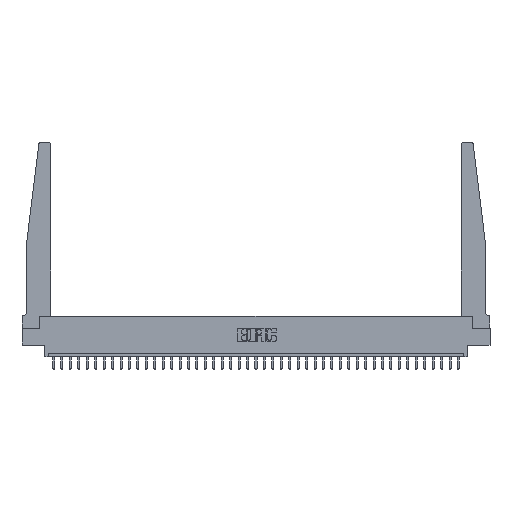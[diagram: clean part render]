
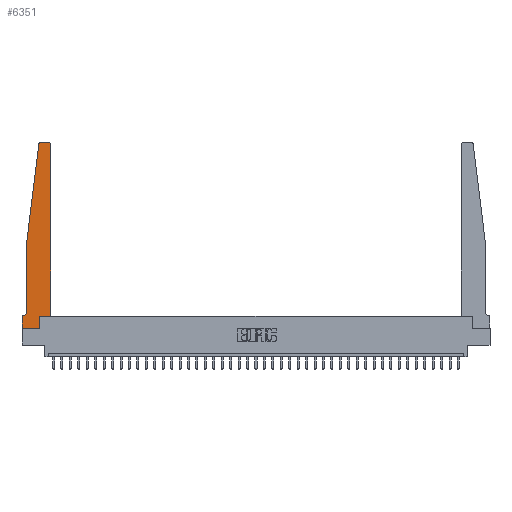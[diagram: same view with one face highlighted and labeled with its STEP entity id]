
A CAD part, top view. The second image highlights one B-rep face of the part: STEP entity #6351.
In plain terms, the highlighted planar face has unit normal (0, 0, 1).
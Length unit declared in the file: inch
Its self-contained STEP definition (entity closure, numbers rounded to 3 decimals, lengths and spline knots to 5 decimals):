
#973 = VERTEX_POINT ( 'NONE', #13403 ) ;
#2054 = EDGE_CURVE ( 'NONE', #10058, #14015, #32561, .T. ) ;
#2239 = EDGE_CURVE ( 'NONE', #14015, #20525, #28684, .T. ) ;
#2964 = CARTESIAN_POINT ( 'NONE',  ( 0.425, 0.18, 0.37 ) ) ;
#3922 = CIRCLE ( 'NONE', #4487, 0.03 ) ;
#4487 = AXIS2_PLACEMENT_3D ( 'NONE', #12611, #20382, #20739 ) ;
#4509 = AXIS2_PLACEMENT_3D ( 'NONE', #16735, #30331, #5961 ) ;
#4637 = VECTOR ( 'NONE', #10681, 39.37008 ) ;
#5899 = ORIENTED_EDGE ( 'NONE', *, *, #2054, .T. ) ;
#5961 = DIRECTION ( 'NONE',  ( 1., 0., 0. ) ) ;
#6138 = AXIS2_PLACEMENT_3D ( 'NONE', #26062, #28873, #11899 ) ;
#6351 = ADVANCED_FACE ( 'NONE', ( #18101 ), #31167, .T. ) ;
#6435 = VERTEX_POINT ( 'NONE', #12617 ) ;
#6748 = DIRECTION ( 'NONE',  ( 0., 1., 0. ) ) ;
#7645 = DIRECTION ( 'NONE',  ( 1., 0., 0. ) ) ;
#8675 = EDGE_CURVE ( 'NONE', #973, #26831, #27180, .T. ) ;
#8802 = EDGE_CURVE ( 'NONE', #9915, #18805, #3922, .T. ) ;
#9577 = ORIENTED_EDGE ( 'NONE', *, *, #8802, .T. ) ;
#9644 = CIRCLE ( 'NONE', #21502, 0.05 ) ;
#9915 = VERTEX_POINT ( 'NONE', #11609 ) ;
#10058 = VERTEX_POINT ( 'NONE', #22925 ) ;
#10526 = ORIENTED_EDGE ( 'NONE', *, *, #13420, .T. ) ;
#10645 = ORIENTED_EDGE ( 'NONE', *, *, #27091, .T. ) ;
#10681 = DIRECTION ( 'NONE',  ( 0., -1., 0. ) ) ;
#10792 = VECTOR ( 'NONE', #28868, 39.37008 ) ;
#11255 = CIRCLE ( 'NONE', #4509, 0.03 ) ;
#11312 = EDGE_CURVE ( 'NONE', #31281, #30662, #16021, .T. ) ;
#11443 = CARTESIAN_POINT ( 'NONE',  ( 0.065, 1.25, 0.37 ) ) ;
#11609 = CARTESIAN_POINT ( 'NONE',  ( 0.425, 2.72, 0.37 ) ) ;
#11742 = LINE ( 'NONE', #28026, #25545 ) ;
#11899 = DIRECTION ( 'NONE',  ( 1., 0., 0. ) ) ;
#11910 = DIRECTION ( 'NONE',  ( -1., 0., 0. ) ) ;
#12081 = DIRECTION ( 'NONE',  ( 0., 0., -1. ) ) ;
#12142 = VERTEX_POINT ( 'NONE', #29181 ) ;
#12611 = CARTESIAN_POINT ( 'NONE',  ( 0.395, 2.72, 0.37 ) ) ;
#12617 = CARTESIAN_POINT ( 'NONE',  ( 0.015, 0.1875, 0.37 ) ) ;
#13403 = CARTESIAN_POINT ( 'NONE',  ( 0.2605, 0.18, 0.37 ) ) ;
#13420 = EDGE_CURVE ( 'NONE', #6435, #10058, #17910, .T. ) ;
#14015 = VERTEX_POINT ( 'NONE', #24927 ) ;
#14018 = CARTESIAN_POINT ( 'NONE',  ( 0., 0., 0.37 ) ) ;
#14509 = CARTESIAN_POINT ( 'NONE',  ( 0.2605, 0., 0.37 ) ) ;
#14522 = CARTESIAN_POINT ( 'NONE',  ( 0.2605, 0.18, 0.37 ) ) ;
#14621 = VECTOR ( 'NONE', #16326, 39.37008 ) ;
#15306 = CARTESIAN_POINT ( 'NONE',  ( 0.065, 1.25, 0.37 ) ) ;
#15410 = CARTESIAN_POINT ( 'NONE',  ( 0.24675, 2.72367, 0.37 ) ) ;
#16021 = LINE ( 'NONE', #24165, #4637 ) ;
#16326 = DIRECTION ( 'NONE',  ( 0., -1., 0. ) ) ;
#16675 = EDGE_LOOP ( 'NONE', ( #10645, #28558, #20819, #27035, #30135, #10526, #5899, #21959, #34791, #30148, #29580, #9577 ) ) ;
#16735 = CARTESIAN_POINT ( 'NONE',  ( 0.27653, 2.72, 0.37 ) ) ;
#17910 = LINE ( 'NONE', #28699, #10792 ) ;
#18101 = FACE_OUTER_BOUND ( 'NONE', #16675, .T. ) ;
#18251 = CARTESIAN_POINT ( 'NONE',  ( 0.065, 0.2375, 0.37 ) ) ;
#18805 = VERTEX_POINT ( 'NONE', #31724 ) ;
#18861 = EDGE_CURVE ( 'NONE', #33782, #31281, #28737, .T. ) ;
#19688 = CARTESIAN_POINT ( 'NONE',  ( 0.015, 0.2375, 0.37 ) ) ;
#19974 = CARTESIAN_POINT ( 'NONE',  ( 0.425, 0.18, 0.37 ) ) ;
#20382 = DIRECTION ( 'NONE',  ( 0., 0., 1. ) ) ;
#20525 = VERTEX_POINT ( 'NONE', #14509 ) ;
#20739 = DIRECTION ( 'NONE',  ( 1., 0., 0. ) ) ;
#20819 = ORIENTED_EDGE ( 'NONE', *, *, #18861, .T. ) ;
#21039 = VECTOR ( 'NONE', #6748, 39.37008 ) ;
#21502 = AXIS2_PLACEMENT_3D ( 'NONE', #19688, #12081, #30645 ) ;
#21959 = ORIENTED_EDGE ( 'NONE', *, *, #2239, .T. ) ;
#22439 = LINE ( 'NONE', #32677, #32826 ) ;
#22634 = EDGE_CURVE ( 'NONE', #12142, #33782, #11255, .T. ) ;
#22925 = CARTESIAN_POINT ( 'NONE',  ( 0., 0.1875, 0.37 ) ) ;
#23460 = DIRECTION ( 'NONE',  ( -0.122, -0.992, 0. ) ) ;
#24165 = CARTESIAN_POINT ( 'NONE',  ( 0.065, 1.25, 0.37 ) ) ;
#24927 = CARTESIAN_POINT ( 'NONE',  ( 0., 0., 0.37 ) ) ;
#25545 = VECTOR ( 'NONE', #11910, 39.37008 ) ;
#26062 = CARTESIAN_POINT ( 'NONE',  ( 0., 0.1875, 0.37 ) ) ;
#26433 = EDGE_CURVE ( 'NONE', #20525, #973, #30780, .T. ) ;
#26752 = EDGE_CURVE ( 'NONE', #26831, #9915, #22439, .T. ) ;
#26831 = VERTEX_POINT ( 'NONE', #19974 ) ;
#27035 = ORIENTED_EDGE ( 'NONE', *, *, #11312, .T. ) ;
#27091 = EDGE_CURVE ( 'NONE', #18805, #12142, #11742, .T. ) ;
#27180 = LINE ( 'NONE', #2964, #27630 ) ;
#27575 = DIRECTION ( 'NONE',  ( 0., 1., 0. ) ) ;
#27630 = VECTOR ( 'NONE', #32796, 39.37008 ) ;
#27663 = VECTOR ( 'NONE', #7645, 39.37008 ) ;
#28026 = CARTESIAN_POINT ( 'NONE',  ( 0.25, 2.75, 0.37 ) ) ;
#28558 = ORIENTED_EDGE ( 'NONE', *, *, #22634, .T. ) ;
#28684 = LINE ( 'NONE', #34322, #27663 ) ;
#28699 = CARTESIAN_POINT ( 'NONE',  ( 0.065, 0.1875, 0.37 ) ) ;
#28737 = LINE ( 'NONE', #15306, #34309 ) ;
#28868 = DIRECTION ( 'NONE',  ( -1., 0., 0. ) ) ;
#28873 = DIRECTION ( 'NONE',  ( 0., 0., 1. ) ) ;
#29181 = CARTESIAN_POINT ( 'NONE',  ( 0.27653, 2.75, 0.37 ) ) ;
#29580 = ORIENTED_EDGE ( 'NONE', *, *, #26752, .T. ) ;
#30135 = ORIENTED_EDGE ( 'NONE', *, *, #33103, .T. ) ;
#30148 = ORIENTED_EDGE ( 'NONE', *, *, #8675, .T. ) ;
#30331 = DIRECTION ( 'NONE',  ( 0., 0., 1. ) ) ;
#30645 = DIRECTION ( 'NONE',  ( -1., 0., 0. ) ) ;
#30662 = VERTEX_POINT ( 'NONE', #18251 ) ;
#30780 = LINE ( 'NONE', #14522, #21039 ) ;
#31167 = PLANE ( 'NONE',  #6138 ) ;
#31281 = VERTEX_POINT ( 'NONE', #11443 ) ;
#31724 = CARTESIAN_POINT ( 'NONE',  ( 0.395, 2.75, 0.37 ) ) ;
#32561 = LINE ( 'NONE', #14018, #14621 ) ;
#32677 = CARTESIAN_POINT ( 'NONE',  ( 0.425, 0.18, 0.37 ) ) ;
#32796 = DIRECTION ( 'NONE',  ( 1., 0., 0. ) ) ;
#32826 = VECTOR ( 'NONE', #27575, 39.37008 ) ;
#33103 = EDGE_CURVE ( 'NONE', #30662, #6435, #9644, .T. ) ;
#33782 = VERTEX_POINT ( 'NONE', #15410 ) ;
#34309 = VECTOR ( 'NONE', #23460, 39.37008 ) ;
#34322 = CARTESIAN_POINT ( 'NONE',  ( 0., 0., 0.37 ) ) ;
#34791 = ORIENTED_EDGE ( 'NONE', *, *, #26433, .T. ) ;
